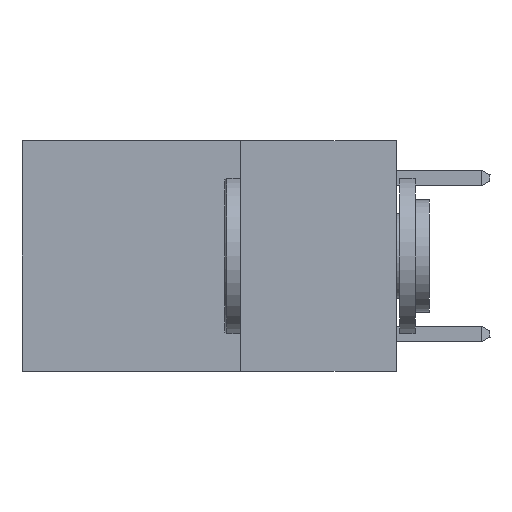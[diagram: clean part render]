
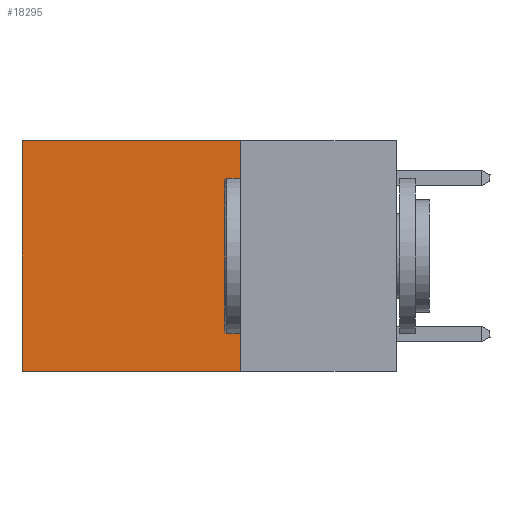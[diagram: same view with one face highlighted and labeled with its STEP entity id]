
A CAD part, left-side view. The second image highlights one B-rep face of the part: STEP entity #18295.
In plain terms, the highlighted planar face has unit normal (-1, 0, 0).
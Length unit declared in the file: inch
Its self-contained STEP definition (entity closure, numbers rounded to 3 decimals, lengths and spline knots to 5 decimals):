
#1110 = EDGE_CURVE ( 'NONE', #12496, #2152, #19387, .T. ) ;
#1149 = EDGE_LOOP ( 'NONE', ( #6155, #6105, #4546, #20110 ) ) ;
#1618 = DIRECTION ( 'NONE',  ( 0., 0., -1. ) ) ;
#1792 = VECTOR ( 'NONE', #6997, 39.37008 ) ;
#1800 = DIRECTION ( 'NONE',  ( 0., 0., -1. ) ) ;
#1997 = CARTESIAN_POINT ( 'NONE',  ( 0.2625, 0.6, 0. ) ) ;
#2152 = VERTEX_POINT ( 'NONE', #1997 ) ;
#2722 = VECTOR ( 'NONE', #10818, 39.37008 ) ;
#3568 = PLANE ( 'NONE',  #4221 ) ;
#4221 = AXIS2_PLACEMENT_3D ( 'NONE', #19643, #12244, #1618 ) ;
#4546 = ORIENTED_EDGE ( 'NONE', *, *, #6491, .F. ) ;
#5769 = LINE ( 'NONE', #21854, #11852 ) ;
#6105 = ORIENTED_EDGE ( 'NONE', *, *, #7194, .F. ) ;
#6155 = ORIENTED_EDGE ( 'NONE', *, *, #12188, .T. ) ;
#6491 = EDGE_CURVE ( 'NONE', #12496, #16416, #15568, .T. ) ;
#6997 = DIRECTION ( 'NONE',  ( 0., 1., 0. ) ) ;
#7194 = EDGE_CURVE ( 'NONE', #16416, #8094, #5769, .T. ) ;
#8094 = VERTEX_POINT ( 'NONE', #12665 ) ;
#10702 = CARTESIAN_POINT ( 'NONE',  ( 0.2625, 0.6, 0. ) ) ;
#10818 = DIRECTION ( 'NONE',  ( 0., 0., -1. ) ) ;
#11852 = VECTOR ( 'NONE', #14690, 39.37008 ) ;
#12188 = EDGE_CURVE ( 'NONE', #2152, #8094, #19380, .T. ) ;
#12244 = DIRECTION ( 'NONE',  ( 1., 0., 0. ) ) ;
#12496 = VERTEX_POINT ( 'NONE', #13919 ) ;
#12665 = CARTESIAN_POINT ( 'NONE',  ( 0.2625, 0.6, -0.37 ) ) ;
#13919 = CARTESIAN_POINT ( 'NONE',  ( 0.2625, 0.25, 0. ) ) ;
#14690 = DIRECTION ( 'NONE',  ( 0., 1., 0. ) ) ;
#15568 = LINE ( 'NONE', #15787, #16633 ) ;
#15787 = CARTESIAN_POINT ( 'NONE',  ( 0.2625, 0.25, 0. ) ) ;
#15809 = CARTESIAN_POINT ( 'NONE',  ( 0.2625, 0.25, 0. ) ) ;
#16416 = VERTEX_POINT ( 'NONE', #19523 ) ;
#16633 = VECTOR ( 'NONE', #1800, 39.37008 ) ;
#18295 = ADVANCED_FACE ( 'NONE', ( #21370 ), #3568, .F. ) ;
#19380 = LINE ( 'NONE', #10702, #2722 ) ;
#19387 = LINE ( 'NONE', #15809, #1792 ) ;
#19523 = CARTESIAN_POINT ( 'NONE',  ( 0.2625, 0.25, -0.37 ) ) ;
#19643 = CARTESIAN_POINT ( 'NONE',  ( 0.2625, 0.25, 0. ) ) ;
#20110 = ORIENTED_EDGE ( 'NONE', *, *, #1110, .T. ) ;
#21370 = FACE_OUTER_BOUND ( 'NONE', #1149, .T. ) ;
#21854 = CARTESIAN_POINT ( 'NONE',  ( 0.2625, 0.25, -0.37 ) ) ;
